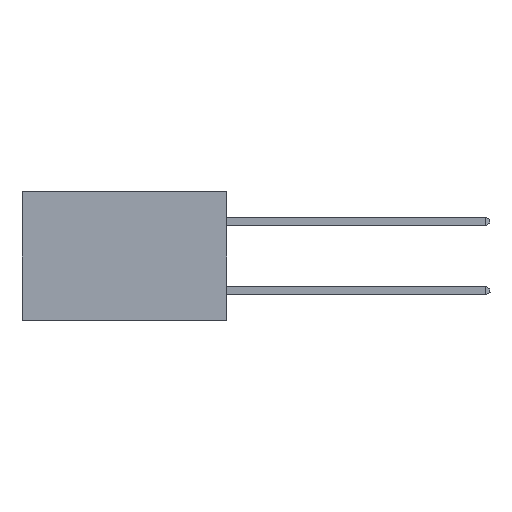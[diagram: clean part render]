
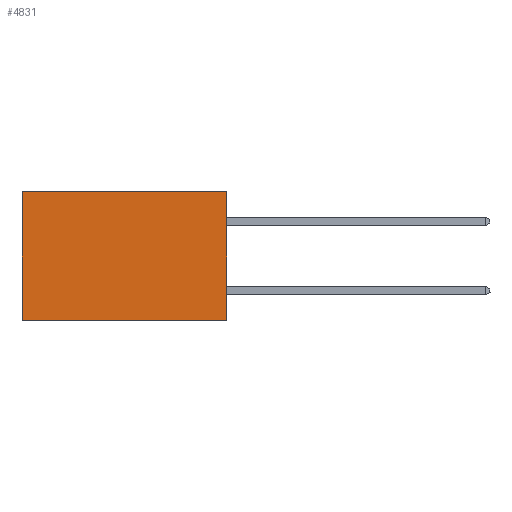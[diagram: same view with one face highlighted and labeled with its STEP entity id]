
A CAD part, left-side view. The second image highlights one B-rep face of the part: STEP entity #4831.
In plain terms, the highlighted planar face has unit normal (-1, 0, 0).
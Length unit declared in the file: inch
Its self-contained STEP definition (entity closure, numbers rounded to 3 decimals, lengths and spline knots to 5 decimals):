
#32 = CARTESIAN_POINT ( 'NONE',  ( 0.277, 0.59, -0.37 ) ) ;
#619 = VECTOR ( 'NONE', #14409, 39.37008 ) ;
#3737 = VERTEX_POINT ( 'NONE', #22125 ) ;
#4831 = ADVANCED_FACE ( 'NONE', ( #26739 ), #19539, .F. ) ;
#5100 = EDGE_CURVE ( 'NONE', #3737, #27942, #13721, .T. ) ;
#5289 = VECTOR ( 'NONE', #20315, 39.37008 ) ;
#5665 = CARTESIAN_POINT ( 'NONE',  ( 0.277, 0.59, -0.37 ) ) ;
#8752 = AXIS2_PLACEMENT_3D ( 'NONE', #28291, #18843, #18628 ) ;
#10221 = CARTESIAN_POINT ( 'NONE',  ( 0.277, 0.59, 0. ) ) ;
#11924 = VERTEX_POINT ( 'NONE', #5665 ) ;
#13144 = VECTOR ( 'NONE', #20506, 39.37008 ) ;
#13183 = ORIENTED_EDGE ( 'NONE', *, *, #29369, .T. ) ;
#13721 = LINE ( 'NONE', #23203, #5289 ) ;
#14229 = DIRECTION ( 'NONE',  ( 0., 1., 0. ) ) ;
#14409 = DIRECTION ( 'NONE',  ( 0., 1., 0. ) ) ;
#14560 = ORIENTED_EDGE ( 'NONE', *, *, #28110, .T. ) ;
#14608 = EDGE_CURVE ( 'NONE', #27942, #11924, #19092, .T. ) ;
#17701 = VERTEX_POINT ( 'NONE', #10221 ) ;
#18157 = ORIENTED_EDGE ( 'NONE', *, *, #14608, .F. ) ;
#18294 = VECTOR ( 'NONE', #14229, 39.37008 ) ;
#18628 = DIRECTION ( 'NONE',  ( 0., 0., -1. ) ) ;
#18843 = DIRECTION ( 'NONE',  ( 1., 0., 0. ) ) ;
#19092 = LINE ( 'NONE', #26789, #18294 ) ;
#19539 = PLANE ( 'NONE',  #8752 ) ;
#20315 = DIRECTION ( 'NONE',  ( 0., 0., -1. ) ) ;
#20506 = DIRECTION ( 'NONE',  ( 0., 0., -1. ) ) ;
#20998 = LINE ( 'NONE', #26973, #619 ) ;
#21830 = ORIENTED_EDGE ( 'NONE', *, *, #5100, .F. ) ;
#22125 = CARTESIAN_POINT ( 'NONE',  ( 0.277, 0., 0. ) ) ;
#22758 = EDGE_LOOP ( 'NONE', ( #14560, #18157, #21830, #13183 ) ) ;
#23203 = CARTESIAN_POINT ( 'NONE',  ( 0.277, 0., -0.37 ) ) ;
#26558 = LINE ( 'NONE', #32, #13144 ) ;
#26739 = FACE_OUTER_BOUND ( 'NONE', #22758, .T. ) ;
#26789 = CARTESIAN_POINT ( 'NONE',  ( 0.277, 0., -0.37 ) ) ;
#26973 = CARTESIAN_POINT ( 'NONE',  ( 0.277, 0., 0. ) ) ;
#27942 = VERTEX_POINT ( 'NONE', #32405 ) ;
#28110 = EDGE_CURVE ( 'NONE', #17701, #11924, #26558, .T. ) ;
#28291 = CARTESIAN_POINT ( 'NONE',  ( 0.277, 0., -0.37 ) ) ;
#29369 = EDGE_CURVE ( 'NONE', #3737, #17701, #20998, .T. ) ;
#32405 = CARTESIAN_POINT ( 'NONE',  ( 0.277, 0., -0.37 ) ) ;
